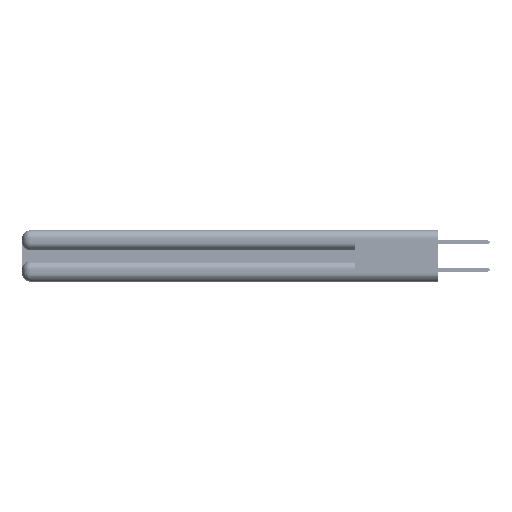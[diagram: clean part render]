
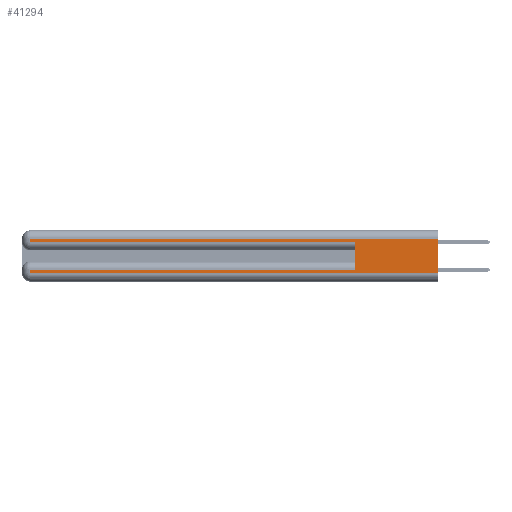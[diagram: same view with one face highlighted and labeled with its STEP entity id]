
A CAD part, left-side view. The second image highlights one B-rep face of the part: STEP entity #41294.
In plain terms, the highlighted planar face has unit normal (-1, 0, 0).
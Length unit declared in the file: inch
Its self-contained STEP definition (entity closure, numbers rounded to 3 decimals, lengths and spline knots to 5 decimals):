
#1237 = CARTESIAN_POINT ( 'NONE',  ( 0., 0.6, 0.085 ) ) ;
#4118 = LINE ( 'NONE', #10464, #36721 ) ;
#4586 = VERTEX_POINT ( 'NONE', #42506 ) ;
#4854 = ORIENTED_EDGE ( 'NONE', *, *, #40380, .F. ) ;
#5320 = DIRECTION ( 'NONE',  ( 0., 1., 0. ) ) ;
#5692 = PLANE ( 'NONE',  #22828 ) ;
#6001 = DIRECTION ( 'NONE',  ( 0., 0., -1. ) ) ;
#6077 = DIRECTION ( 'NONE',  ( 1., 0., 0. ) ) ;
#7006 = LINE ( 'NONE', #52590, #16992 ) ;
#7300 = LINE ( 'NONE', #9508, #27942 ) ;
#8965 = CARTESIAN_POINT ( 'NONE',  ( 0., 0.6, 0.285 ) ) ;
#9508 = CARTESIAN_POINT ( 'NONE',  ( 0., 0.6, 0.145 ) ) ;
#10179 = CARTESIAN_POINT ( 'NONE',  ( 0., 0., 0.085 ) ) ;
#10464 = CARTESIAN_POINT ( 'NONE',  ( 0., 0., 0.37 ) ) ;
#10496 = VERTEX_POINT ( 'NONE', #54446 ) ;
#12566 = VECTOR ( 'NONE', #28316, 39.37008 ) ;
#12828 = EDGE_CURVE ( 'NONE', #41229, #10496, #4118, .T. ) ;
#14031 = VECTOR ( 'NONE', #34503, 39.37008 ) ;
#14491 = FACE_OUTER_BOUND ( 'NONE', #51418, .T. ) ;
#14543 = LINE ( 'NONE', #54079, #12566 ) ;
#14991 = ORIENTED_EDGE ( 'NONE', *, *, #12828, .F. ) ;
#16992 = VECTOR ( 'NONE', #32326, 39.37008 ) ;
#17867 = VECTOR ( 'NONE', #5320, 39.37008 ) ;
#20767 = VERTEX_POINT ( 'NONE', #24275 ) ;
#20890 = CARTESIAN_POINT ( 'NONE',  ( 0., 2.94, 0.285 ) ) ;
#22075 = ORIENTED_EDGE ( 'NONE', *, *, #46463, .T. ) ;
#22264 = CARTESIAN_POINT ( 'NONE',  ( 0., 0., 0.31 ) ) ;
#22731 = LINE ( 'NONE', #10179, #40639 ) ;
#22828 = AXIS2_PLACEMENT_3D ( 'NONE', #35631, #6077, #31152 ) ;
#23657 = LINE ( 'NONE', #25405, #34330 ) ;
#24275 = CARTESIAN_POINT ( 'NONE',  ( 0., 2.94, 0.31 ) ) ;
#24792 = EDGE_CURVE ( 'NONE', #45063, #4586, #7006, .T. ) ;
#25405 = CARTESIAN_POINT ( 'NONE',  ( 0., 0., 0.285 ) ) ;
#25951 = DIRECTION ( 'NONE',  ( 0., -1., 0. ) ) ;
#26763 = DIRECTION ( 'NONE',  ( 0., 1., 0. ) ) ;
#27088 = EDGE_CURVE ( 'NONE', #20767, #50071, #14543, .T. ) ;
#27942 = VECTOR ( 'NONE', #52064, 39.37008 ) ;
#27948 = EDGE_CURVE ( 'NONE', #41229, #20767, #49081, .T. ) ;
#28316 = DIRECTION ( 'NONE',  ( 0., 0., -1. ) ) ;
#31152 = DIRECTION ( 'NONE',  ( 0., 0., -1. ) ) ;
#31804 = EDGE_CURVE ( 'NONE', #4586, #10496, #39977, .T. ) ;
#32326 = DIRECTION ( 'NONE',  ( 0., 0., -1. ) ) ;
#32904 = ORIENTED_EDGE ( 'NONE', *, *, #27088, .T. ) ;
#34330 = VECTOR ( 'NONE', #25951, 39.37008 ) ;
#34503 = DIRECTION ( 'NONE',  ( 0., -1., 0. ) ) ;
#35553 = ORIENTED_EDGE ( 'NONE', *, *, #24792, .T. ) ;
#35631 = CARTESIAN_POINT ( 'NONE',  ( 0., 0., 0.37 ) ) ;
#35954 = ORIENTED_EDGE ( 'NONE', *, *, #27948, .T. ) ;
#36721 = VECTOR ( 'NONE', #6001, 39.37008 ) ;
#39247 = EDGE_CURVE ( 'NONE', #51022, #45063, #22731, .T. ) ;
#39977 = LINE ( 'NONE', #46536, #14031 ) ;
#40380 = EDGE_CURVE ( 'NONE', #51022, #50274, #7300, .T. ) ;
#40639 = VECTOR ( 'NONE', #26763, 39.37008 ) ;
#40906 = ORIENTED_EDGE ( 'NONE', *, *, #39247, .T. ) ;
#41229 = VERTEX_POINT ( 'NONE', #47137 ) ;
#41294 = ADVANCED_FACE ( 'NONE', ( #14491 ), #5692, .F. ) ;
#42506 = CARTESIAN_POINT ( 'NONE',  ( 0., 2.94, 0.06 ) ) ;
#43103 = CARTESIAN_POINT ( 'NONE',  ( 0., 2.94, 0.085 ) ) ;
#45063 = VERTEX_POINT ( 'NONE', #43103 ) ;
#45864 = ORIENTED_EDGE ( 'NONE', *, *, #31804, .T. ) ;
#46463 = EDGE_CURVE ( 'NONE', #50071, #50274, #23657, .T. ) ;
#46536 = CARTESIAN_POINT ( 'NONE',  ( 0., 0., 0.06 ) ) ;
#47137 = CARTESIAN_POINT ( 'NONE',  ( 0., 0., 0.31 ) ) ;
#49081 = LINE ( 'NONE', #22264, #17867 ) ;
#50071 = VERTEX_POINT ( 'NONE', #20890 ) ;
#50274 = VERTEX_POINT ( 'NONE', #8965 ) ;
#51022 = VERTEX_POINT ( 'NONE', #1237 ) ;
#51418 = EDGE_LOOP ( 'NONE', ( #14991, #35954, #32904, #22075, #4854, #40906, #35553, #45864 ) ) ;
#52064 = DIRECTION ( 'NONE',  ( 0., 0., 1. ) ) ;
#52590 = CARTESIAN_POINT ( 'NONE',  ( 0., 2.94, 0.37 ) ) ;
#54079 = CARTESIAN_POINT ( 'NONE',  ( 0., 2.94, 0.37 ) ) ;
#54446 = CARTESIAN_POINT ( 'NONE',  ( 0., 0., 0.06 ) ) ;
